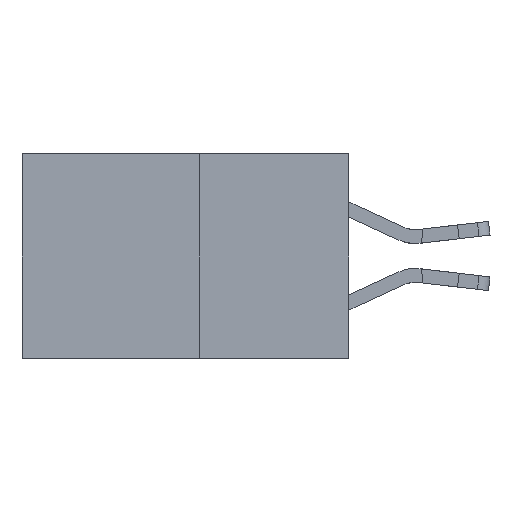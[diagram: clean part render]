
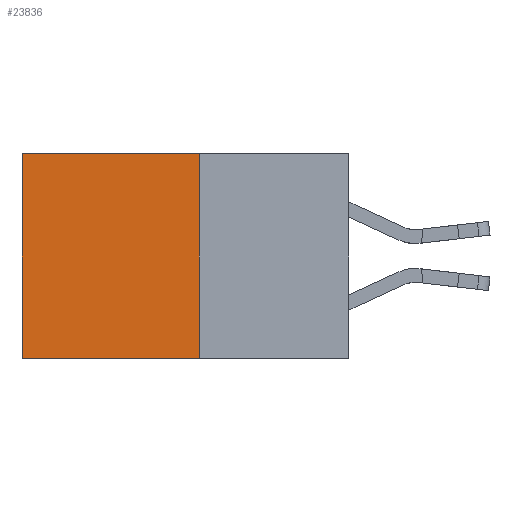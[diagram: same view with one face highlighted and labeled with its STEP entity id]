
A CAD part, left-side view. The second image highlights one B-rep face of the part: STEP entity #23836.
In plain terms, the highlighted planar face has unit normal (-1, 0, 0).
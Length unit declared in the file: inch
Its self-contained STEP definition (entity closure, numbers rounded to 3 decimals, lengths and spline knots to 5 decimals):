
#200 = DIRECTION ( 'NONE',  ( 0., 0., -1. ) ) ;
#2714 = CARTESIAN_POINT ( 'NONE',  ( 0.277, 0.27, -0.37 ) ) ;
#2920 = CARTESIAN_POINT ( 'NONE',  ( 0.277, 0.27, 0. ) ) ;
#2972 = CARTESIAN_POINT ( 'NONE',  ( 0.277, 0.27, 0. ) ) ;
#4082 = VERTEX_POINT ( 'NONE', #12111 ) ;
#5220 = ORIENTED_EDGE ( 'NONE', *, *, #18102, .F. ) ;
#5960 = AXIS2_PLACEMENT_3D ( 'NONE', #10688, #25992, #10802 ) ;
#6762 = LINE ( 'NONE', #18108, #24673 ) ;
#10688 = CARTESIAN_POINT ( 'NONE',  ( 0.277, 0.27, -0.37 ) ) ;
#10802 = DIRECTION ( 'NONE',  ( 0., 0., -1. ) ) ;
#11810 = VERTEX_POINT ( 'NONE', #12644 ) ;
#11938 = LINE ( 'NONE', #2920, #17910 ) ;
#12111 = CARTESIAN_POINT ( 'NONE',  ( 0.277, 0.59, 0. ) ) ;
#12644 = CARTESIAN_POINT ( 'NONE',  ( 0.277, 0.27, -0.37 ) ) ;
#12949 = VERTEX_POINT ( 'NONE', #16842 ) ;
#13217 = DIRECTION ( 'NONE',  ( 0., 1., 0. ) ) ;
#14272 = FACE_OUTER_BOUND ( 'NONE', #19087, .T. ) ;
#16842 = CARTESIAN_POINT ( 'NONE',  ( 0.277, 0.59, -0.37 ) ) ;
#17673 = VERTEX_POINT ( 'NONE', #2972 ) ;
#17910 = VECTOR ( 'NONE', #13217, 39.37008 ) ;
#18102 = EDGE_CURVE ( 'NONE', #17673, #11810, #19405, .T. ) ;
#18108 = CARTESIAN_POINT ( 'NONE',  ( 0.277, 0.59, -0.37 ) ) ;
#18372 = PLANE ( 'NONE',  #5960 ) ;
#19087 = EDGE_LOOP ( 'NONE', ( #23477, #30650, #5220, #26486 ) ) ;
#19405 = LINE ( 'NONE', #27429, #21000 ) ;
#19814 = DIRECTION ( 'NONE',  ( 0., 0., -1. ) ) ;
#21000 = VECTOR ( 'NONE', #19814, 39.37008 ) ;
#23202 = DIRECTION ( 'NONE',  ( 0., 1., 0. ) ) ;
#23340 = LINE ( 'NONE', #2714, #31666 ) ;
#23477 = ORIENTED_EDGE ( 'NONE', *, *, #30808, .T. ) ;
#23836 = ADVANCED_FACE ( 'NONE', ( #14272 ), #18372, .F. ) ;
#24559 = EDGE_CURVE ( 'NONE', #17673, #4082, #11938, .T. ) ;
#24673 = VECTOR ( 'NONE', #200, 39.37008 ) ;
#25992 = DIRECTION ( 'NONE',  ( 1., 0., 0. ) ) ;
#26140 = EDGE_CURVE ( 'NONE', #11810, #12949, #23340, .T. ) ;
#26486 = ORIENTED_EDGE ( 'NONE', *, *, #24559, .T. ) ;
#27429 = CARTESIAN_POINT ( 'NONE',  ( 0.277, 0.27, -0.37 ) ) ;
#30650 = ORIENTED_EDGE ( 'NONE', *, *, #26140, .F. ) ;
#30808 = EDGE_CURVE ( 'NONE', #4082, #12949, #6762, .T. ) ;
#31666 = VECTOR ( 'NONE', #23202, 39.37008 ) ;
